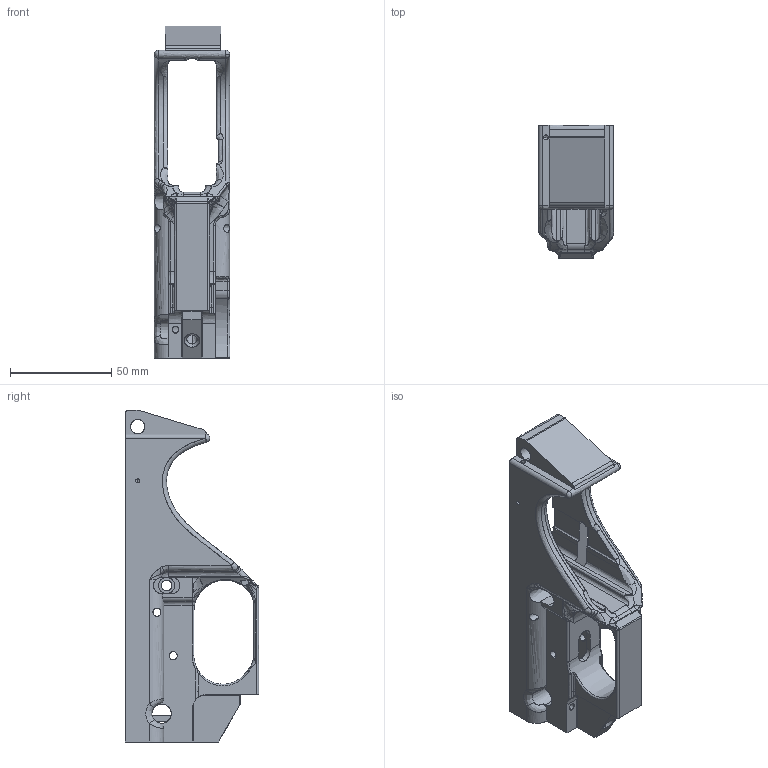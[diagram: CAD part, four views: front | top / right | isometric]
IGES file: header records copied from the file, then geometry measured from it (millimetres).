
Start section: SolidWorks IGES file using analytic representation for surfaces
Global section: file name: Hermes_v1.4_Front.IGS; native system: SolidWorks 2015; preprocessor: SolidWorks 2015; author: WarFairy; date: 150521.101204; units: inch
Bounding box: 37.13 x 65.79 x 163.69 mm (x, y, z)
Surface area: 40311.9 mm2 (no closed solid volume)
Topology: 0 solids, 0 shells, 395 faces, 4870 edges, 4850 vertices
Faces by surface type: bspline 236, revolution 159
